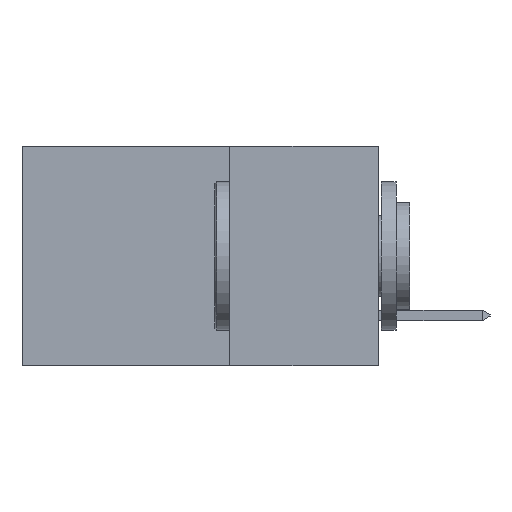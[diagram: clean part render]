
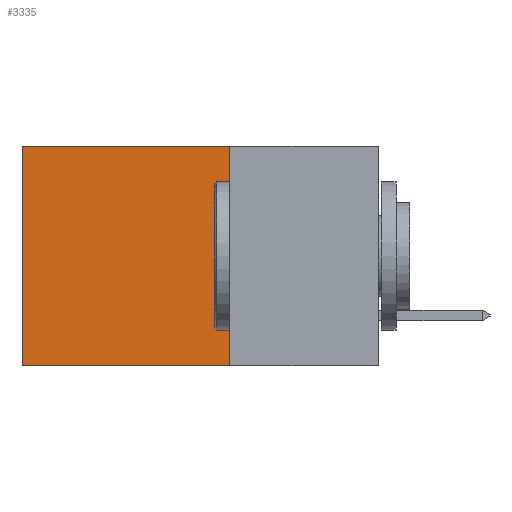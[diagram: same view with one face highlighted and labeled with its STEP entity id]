
A CAD part, left-side view. The second image highlights one B-rep face of the part: STEP entity #3335.
In plain terms, the highlighted planar face has unit normal (-1, 0, 0).
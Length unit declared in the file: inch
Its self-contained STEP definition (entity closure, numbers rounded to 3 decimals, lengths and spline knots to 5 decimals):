
#1009 = LINE ( 'NONE', #1773, #9486 ) ;
#1173 = EDGE_CURVE ( 'NONE', #3924, #12077, #7552, .T. ) ;
#1285 = CARTESIAN_POINT ( 'NONE',  ( 0.2615, 0.25, -0.37 ) ) ;
#1324 = CARTESIAN_POINT ( 'NONE',  ( 0.2615, 0.25, -0.37 ) ) ;
#1764 = EDGE_LOOP ( 'NONE', ( #3104, #13285, #10685, #6144 ) ) ;
#1773 = CARTESIAN_POINT ( 'NONE',  ( 0.2615, 0.25, 0. ) ) ;
#2733 = DIRECTION ( 'NONE',  ( 0., 1., 0. ) ) ;
#3104 = ORIENTED_EDGE ( 'NONE', *, *, #1173, .T. ) ;
#3266 = LINE ( 'NONE', #1324, #11164 ) ;
#3335 = ADVANCED_FACE ( 'NONE', ( #5838 ), #5857, .F. ) ;
#3584 = DIRECTION ( 'NONE',  ( 0., 1., 0. ) ) ;
#3716 = VERTEX_POINT ( 'NONE', #1285 ) ;
#3924 = VERTEX_POINT ( 'NONE', #9236 ) ;
#4271 = DIRECTION ( 'NONE',  ( 0., 0., -1. ) ) ;
#4436 = VECTOR ( 'NONE', #5999, 39.37008 ) ;
#4543 = CARTESIAN_POINT ( 'NONE',  ( 0.2615, 0.25, -0.37 ) ) ;
#4857 = EDGE_CURVE ( 'NONE', #6992, #3716, #5787, .T. ) ;
#5625 = DIRECTION ( 'NONE',  ( 0., 0., -1. ) ) ;
#5629 = DIRECTION ( 'NONE',  ( 1., 0., 0. ) ) ;
#5637 = EDGE_CURVE ( 'NONE', #6992, #3924, #1009, .T. ) ;
#5665 = CARTESIAN_POINT ( 'NONE',  ( 0.2615, 0.25, -0.37 ) ) ;
#5787 = LINE ( 'NONE', #4543, #10894 ) ;
#5817 = CARTESIAN_POINT ( 'NONE',  ( 0.2615, 0.6, -0.37 ) ) ;
#5838 = FACE_OUTER_BOUND ( 'NONE', #1764, .T. ) ;
#5857 = PLANE ( 'NONE',  #8975 ) ;
#5999 = DIRECTION ( 'NONE',  ( 0., 0., -1. ) ) ;
#6144 = ORIENTED_EDGE ( 'NONE', *, *, #5637, .T. ) ;
#6992 = VERTEX_POINT ( 'NONE', #7427 ) ;
#7427 = CARTESIAN_POINT ( 'NONE',  ( 0.2615, 0.25, 0. ) ) ;
#7552 = LINE ( 'NONE', #5817, #4436 ) ;
#8975 = AXIS2_PLACEMENT_3D ( 'NONE', #5665, #5629, #5625 ) ;
#9236 = CARTESIAN_POINT ( 'NONE',  ( 0.2615, 0.6, 0. ) ) ;
#9486 = VECTOR ( 'NONE', #2733, 39.37008 ) ;
#10685 = ORIENTED_EDGE ( 'NONE', *, *, #4857, .F. ) ;
#10894 = VECTOR ( 'NONE', #4271, 39.37008 ) ;
#11164 = VECTOR ( 'NONE', #3584, 39.37008 ) ;
#11607 = CARTESIAN_POINT ( 'NONE',  ( 0.2615, 0.6, -0.37 ) ) ;
#12077 = VERTEX_POINT ( 'NONE', #11607 ) ;
#12722 = EDGE_CURVE ( 'NONE', #3716, #12077, #3266, .T. ) ;
#13285 = ORIENTED_EDGE ( 'NONE', *, *, #12722, .F. ) ;
